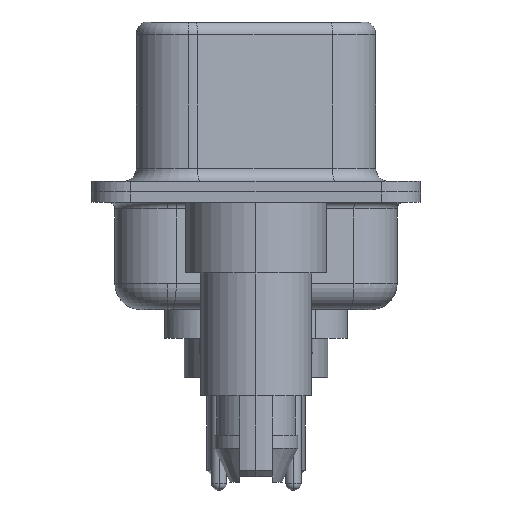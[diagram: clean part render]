
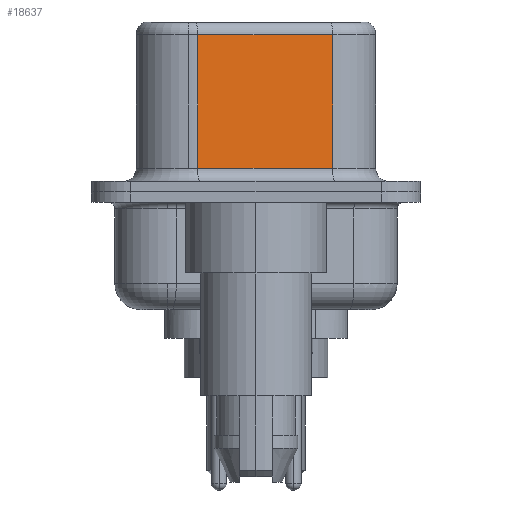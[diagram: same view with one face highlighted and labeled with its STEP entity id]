
A CAD part, left-side view. The second image highlights one B-rep face of the part: STEP entity #18637.
In plain terms, the highlighted planar face has unit normal (-0.985, -0.174, 0).
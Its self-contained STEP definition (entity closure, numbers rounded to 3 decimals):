
#56 = DIRECTION ( 'NONE',  ( 0., 0., -1. ) ) ;
#63 = CARTESIAN_POINT ( 'NONE',  ( 4.58, -2.927, 6.52 ) ) ;
#1401 = LINE ( 'NONE', #7755, #8791 ) ;
#1560 = DIRECTION ( 'NONE',  ( -0.174, 0.985, 0. ) ) ;
#1728 = ORIENTED_EDGE ( 'NONE', *, *, #14088, .F. ) ;
#2906 = LINE ( 'NONE', #9981, #15968 ) ;
#3074 = VERTEX_POINT ( 'NONE', #15833 ) ;
#3471 = LINE ( 'NONE', #12718, #15675 ) ;
#3905 = DIRECTION ( 'NONE',  ( 0.174, -0.985, 0. ) ) ;
#4037 = CARTESIAN_POINT ( 'NONE',  ( 4.58, -2.927, 0.9 ) ) ;
#4940 = CARTESIAN_POINT ( 'NONE',  ( 3.67, 2.233, 0.9 ) ) ;
#7448 = PLANE ( 'NONE',  #9489 ) ;
#7755 = CARTESIAN_POINT ( 'NONE',  ( 4.58, -2.927, 6.02 ) ) ;
#8791 = VECTOR ( 'NONE', #9249, 1000. ) ;
#9249 = DIRECTION ( 'NONE',  ( -0.174, 0.985, 0. ) ) ;
#9489 = AXIS2_PLACEMENT_3D ( 'NONE', #63, #10404, #1560 ) ;
#9981 = CARTESIAN_POINT ( 'NONE',  ( 3.67, 2.233, 6.52 ) ) ;
#10356 = EDGE_CURVE ( 'NONE', #3074, #10700, #2906, .T. ) ;
#10404 = DIRECTION ( 'NONE',  ( 0.985, 0.174, 0. ) ) ;
#10551 = LINE ( 'NONE', #17747, #17940 ) ;
#10700 = VERTEX_POINT ( 'NONE', #4940 ) ;
#11073 = EDGE_LOOP ( 'NONE', ( #1728, #11258, #11667, #14478 ) ) ;
#11258 = ORIENTED_EDGE ( 'NONE', *, *, #11754, .T. ) ;
#11317 = VERTEX_POINT ( 'NONE', #14268 ) ;
#11667 = ORIENTED_EDGE ( 'NONE', *, *, #10356, .T. ) ;
#11754 = EDGE_CURVE ( 'NONE', #11317, #3074, #1401, .T. ) ;
#12507 = EDGE_CURVE ( 'NONE', #10700, #12617, #3471, .T. ) ;
#12617 = VERTEX_POINT ( 'NONE', #4037 ) ;
#12718 = CARTESIAN_POINT ( 'NONE',  ( 4.58, -2.927, 0.9 ) ) ;
#14088 = EDGE_CURVE ( 'NONE', #11317, #12617, #10551, .T. ) ;
#14268 = CARTESIAN_POINT ( 'NONE',  ( 4.58, -2.927, 6.02 ) ) ;
#14478 = ORIENTED_EDGE ( 'NONE', *, *, #12507, .T. ) ;
#15675 = VECTOR ( 'NONE', #3905, 1000. ) ;
#15833 = CARTESIAN_POINT ( 'NONE',  ( 3.67, 2.233, 6.02 ) ) ;
#15968 = VECTOR ( 'NONE', #17322, 1000. ) ;
#17322 = DIRECTION ( 'NONE',  ( 0., 0., -1. ) ) ;
#17747 = CARTESIAN_POINT ( 'NONE',  ( 4.58, -2.927, 6.52 ) ) ;
#17940 = VECTOR ( 'NONE', #56, 1000. ) ;
#18637 = ADVANCED_FACE ( 'NONE', ( #18827 ), #7448, .F. ) ;
#18827 = FACE_OUTER_BOUND ( 'NONE', #11073, .T. ) ;
